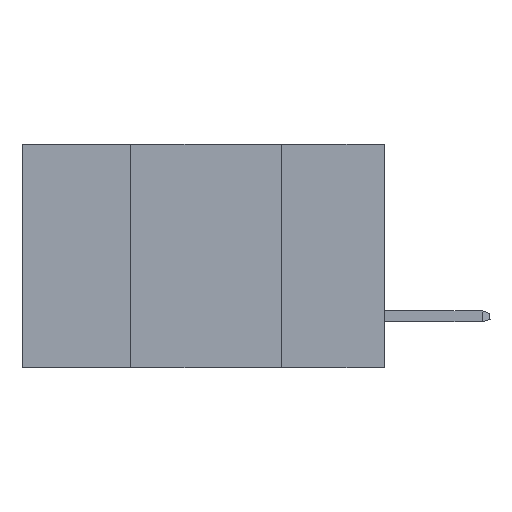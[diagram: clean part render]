
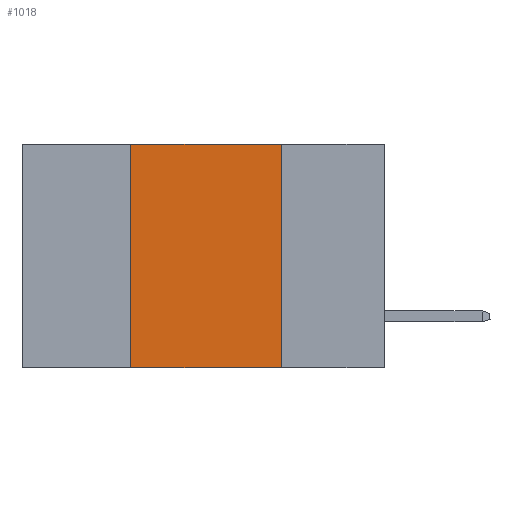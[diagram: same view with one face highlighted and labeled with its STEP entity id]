
A CAD part, left-side view. The second image highlights one B-rep face of the part: STEP entity #1018.
In plain terms, the highlighted planar face has unit normal (-1, 0, 0).
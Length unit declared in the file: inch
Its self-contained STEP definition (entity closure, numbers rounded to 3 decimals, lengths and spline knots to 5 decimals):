
#29 = LINE ( 'NONE', #18075, #12273 ) ;
#347 = DIRECTION ( 'NONE',  ( 0., 0., -1. ) ) ;
#1018 = ADVANCED_FACE ( 'NONE', ( #12093 ), #12164, .F. ) ;
#2738 = ORIENTED_EDGE ( 'NONE', *, *, #4095, .F. ) ;
#2885 = CARTESIAN_POINT ( 'NONE',  ( 0., 0.42, 0. ) ) ;
#3115 = VERTEX_POINT ( 'NONE', #12665 ) ;
#3517 = CARTESIAN_POINT ( 'NONE',  ( 0., 0.6, 0. ) ) ;
#4095 = EDGE_CURVE ( 'NONE', #10710, #16167, #29, .T. ) ;
#4462 = CARTESIAN_POINT ( 'NONE',  ( 0., 0.17, 0. ) ) ;
#5525 = EDGE_CURVE ( 'NONE', #14494, #10710, #7326, .T. ) ;
#5647 = CARTESIAN_POINT ( 'NONE',  ( 0., 0.42, 0. ) ) ;
#6350 = CARTESIAN_POINT ( 'NONE',  ( 0., 0.42, -0.37 ) ) ;
#7196 = LINE ( 'NONE', #11874, #9283 ) ;
#7326 = LINE ( 'NONE', #2885, #17735 ) ;
#7345 = EDGE_LOOP ( 'NONE', ( #9999, #2738, #18468, #14403 ) ) ;
#7705 = DIRECTION ( 'NONE',  ( 1., 0., 0. ) ) ;
#8556 = EDGE_CURVE ( 'NONE', #14494, #3115, #15389, .T. ) ;
#9224 = DIRECTION ( 'NONE',  ( 0., -1., 0. ) ) ;
#9283 = VECTOR ( 'NONE', #19071, 39.37008 ) ;
#9999 = ORIENTED_EDGE ( 'NONE', *, *, #12084, .F. ) ;
#10001 = CARTESIAN_POINT ( 'NONE',  ( 0., 0.6, -0.37 ) ) ;
#10332 = DIRECTION ( 'NONE',  ( 0., -1., 0. ) ) ;
#10710 = VERTEX_POINT ( 'NONE', #5647 ) ;
#11874 = CARTESIAN_POINT ( 'NONE',  ( 0., 0.17, 0. ) ) ;
#12084 = EDGE_CURVE ( 'NONE', #16167, #3115, #7196, .T. ) ;
#12093 = FACE_OUTER_BOUND ( 'NONE', #7345, .T. ) ;
#12164 = PLANE ( 'NONE',  #14124 ) ;
#12172 = VECTOR ( 'NONE', #10332, 39.37008 ) ;
#12273 = VECTOR ( 'NONE', #9224, 39.37008 ) ;
#12665 = CARTESIAN_POINT ( 'NONE',  ( 0., 0.17, -0.37 ) ) ;
#14124 = AXIS2_PLACEMENT_3D ( 'NONE', #3517, #7705, #347 ) ;
#14403 = ORIENTED_EDGE ( 'NONE', *, *, #8556, .T. ) ;
#14494 = VERTEX_POINT ( 'NONE', #6350 ) ;
#15389 = LINE ( 'NONE', #10001, #12172 ) ;
#16167 = VERTEX_POINT ( 'NONE', #4462 ) ;
#16395 = DIRECTION ( 'NONE',  ( 0., 0., 1. ) ) ;
#17735 = VECTOR ( 'NONE', #16395, 39.37008 ) ;
#18075 = CARTESIAN_POINT ( 'NONE',  ( 0., 0.6, 0. ) ) ;
#18468 = ORIENTED_EDGE ( 'NONE', *, *, #5525, .F. ) ;
#19071 = DIRECTION ( 'NONE',  ( 0., 0., -1. ) ) ;
